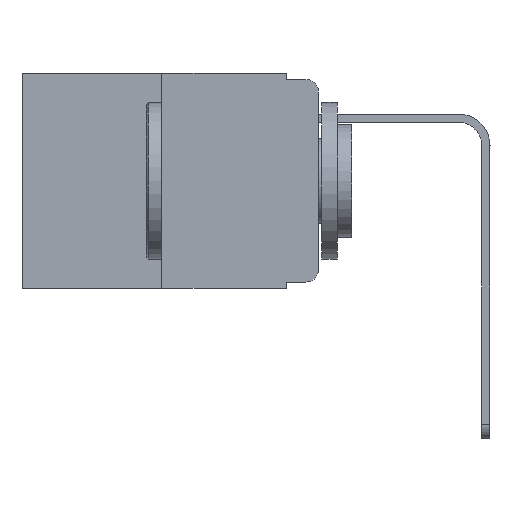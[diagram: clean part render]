
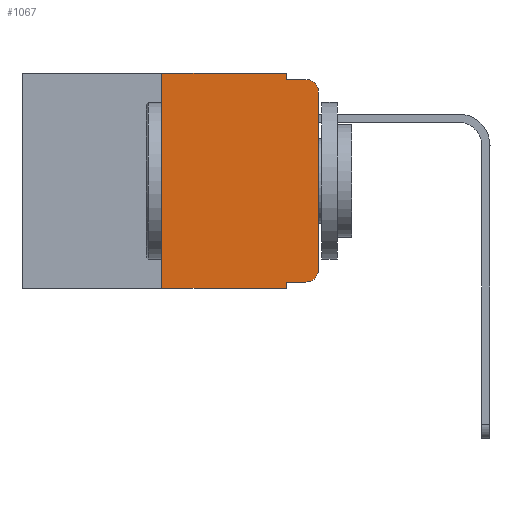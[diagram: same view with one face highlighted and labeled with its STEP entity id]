
A CAD part, left-side view. The second image highlights one B-rep face of the part: STEP entity #1067.
In plain terms, the highlighted planar face has unit normal (-1, 0, 0).
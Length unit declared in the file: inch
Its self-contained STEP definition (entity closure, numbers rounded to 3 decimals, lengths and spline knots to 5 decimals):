
#223 = CARTESIAN_POINT ( 'NONE',  ( 0., 0.051, 0. ) ) ;
#429 = DIRECTION ( 'NONE',  ( 0., 0., 1. ) ) ;
#489 = ORIENTED_EDGE ( 'NONE', *, *, #8777, .T. ) ;
#561 = DIRECTION ( 'NONE',  ( 0., -1., 0. ) ) ;
#603 = VERTEX_POINT ( 'NONE', #2960 ) ;
#658 = DIRECTION ( 'NONE',  ( 0., 0., -1. ) ) ;
#735 = CARTESIAN_POINT ( 'NONE',  ( 0., 0.051, -0.333 ) ) ;
#799 = EDGE_CURVE ( 'NONE', #10643, #1818, #5035, .T. ) ;
#955 = ORIENTED_EDGE ( 'NONE', *, *, #12084, .T. ) ;
#992 = LINE ( 'NONE', #735, #4520 ) ;
#1026 = CARTESIAN_POINT ( 'NONE',  ( 0., 0.02, -0.313 ) ) ;
#1067 = ADVANCED_FACE ( 'NONE', ( #10304 ), #7958, .F. ) ;
#1506 = EDGE_LOOP ( 'NONE', ( #489, #3924, #12947, #4434, #7880, #2469, #955, #7709, #5813, #2844 ) ) ;
#1687 = EDGE_CURVE ( 'NONE', #11537, #8962, #7487, .T. ) ;
#1818 = VERTEX_POINT ( 'NONE', #3817 ) ;
#2043 = DIRECTION ( 'NONE',  ( 0., 0., -1. ) ) ;
#2469 = ORIENTED_EDGE ( 'NONE', *, *, #799, .F. ) ;
#2681 = AXIS2_PLACEMENT_3D ( 'NONE', #11666, #5864, #658 ) ;
#2844 = ORIENTED_EDGE ( 'NONE', *, *, #12909, .T. ) ;
#2897 = DIRECTION ( 'NONE',  ( 0., 0., -1. ) ) ;
#2943 = CARTESIAN_POINT ( 'NONE',  ( 0., 0.473, 0. ) ) ;
#2946 = CARTESIAN_POINT ( 'NONE',  ( 0., 0.473, 0. ) ) ;
#2960 = CARTESIAN_POINT ( 'NONE',  ( 0., 0.051, -0.01 ) ) ;
#3241 = CARTESIAN_POINT ( 'NONE',  ( 0., 0., -0.03 ) ) ;
#3251 = DIRECTION ( 'NONE',  ( -1., 0., 0. ) ) ;
#3274 = LINE ( 'NONE', #10098, #12647 ) ;
#3314 = CARTESIAN_POINT ( 'NONE',  ( 0., 0.051, -0.333 ) ) ;
#3402 = CARTESIAN_POINT ( 'NONE',  ( 0., 0.02, -0.01 ) ) ;
#3679 = DIRECTION ( 'NONE',  ( 0., -1., 0. ) ) ;
#3725 = CARTESIAN_POINT ( 'NONE',  ( 0., 0.051, -0.343 ) ) ;
#3817 = CARTESIAN_POINT ( 'NONE',  ( 0., 0.25, 0. ) ) ;
#3924 = ORIENTED_EDGE ( 'NONE', *, *, #1687, .T. ) ;
#4434 = ORIENTED_EDGE ( 'NONE', *, *, #4542, .F. ) ;
#4520 = VECTOR ( 'NONE', #12689, 39.37008 ) ;
#4542 = EDGE_CURVE ( 'NONE', #12334, #603, #10764, .T. ) ;
#4618 = CIRCLE ( 'NONE', #10205, 0.02 ) ;
#4820 = DIRECTION ( 'NONE',  ( 0., -1., 0. ) ) ;
#4946 = VECTOR ( 'NONE', #561, 39.37008 ) ;
#4997 = EDGE_CURVE ( 'NONE', #8837, #7947, #992, .T. ) ;
#5035 = LINE ( 'NONE', #5432, #12028 ) ;
#5089 = VECTOR ( 'NONE', #4820, 39.37008 ) ;
#5432 = CARTESIAN_POINT ( 'NONE',  ( 0., 0.25, 0. ) ) ;
#5601 = DIRECTION ( 'NONE',  ( 0., 0., -1. ) ) ;
#5721 = LINE ( 'NONE', #6640, #4946 ) ;
#5738 = EDGE_CURVE ( 'NONE', #8837, #12107, #11523, .T. ) ;
#5758 = DIRECTION ( 'NONE',  ( 0., 0., 1. ) ) ;
#5813 = ORIENTED_EDGE ( 'NONE', *, *, #4997, .T. ) ;
#5864 = DIRECTION ( 'NONE',  ( -1., 0., 0. ) ) ;
#6640 = CARTESIAN_POINT ( 'NONE',  ( 0., 0.051, -0.01 ) ) ;
#6788 = CARTESIAN_POINT ( 'NONE',  ( 0., 0.473, -0.343 ) ) ;
#7487 = CIRCLE ( 'NONE', #2681, 0.02 ) ;
#7550 = EDGE_CURVE ( 'NONE', #1818, #12334, #10692, .T. ) ;
#7598 = LINE ( 'NONE', #6788, #10877 ) ;
#7709 = ORIENTED_EDGE ( 'NONE', *, *, #5738, .F. ) ;
#7880 = ORIENTED_EDGE ( 'NONE', *, *, #7550, .F. ) ;
#7947 = VERTEX_POINT ( 'NONE', #12554 ) ;
#7958 = PLANE ( 'NONE',  #8747 ) ;
#8747 = AXIS2_PLACEMENT_3D ( 'NONE', #2943, #8911, #2897 ) ;
#8777 = EDGE_CURVE ( 'NONE', #12714, #11537, #3274, .T. ) ;
#8837 = VERTEX_POINT ( 'NONE', #3314 ) ;
#8890 = VECTOR ( 'NONE', #11678, 39.37008 ) ;
#8911 = DIRECTION ( 'NONE',  ( 1., 0., 0. ) ) ;
#8962 = VERTEX_POINT ( 'NONE', #3402 ) ;
#10098 = CARTESIAN_POINT ( 'NONE',  ( 0., 0., 0. ) ) ;
#10205 = AXIS2_PLACEMENT_3D ( 'NONE', #1026, #3251, #2043 ) ;
#10304 = FACE_OUTER_BOUND ( 'NONE', #1506, .T. ) ;
#10440 = VECTOR ( 'NONE', #5601, 39.37008 ) ;
#10643 = VERTEX_POINT ( 'NONE', #12695 ) ;
#10692 = LINE ( 'NONE', #2946, #5089 ) ;
#10764 = LINE ( 'NONE', #12558, #10440 ) ;
#10877 = VECTOR ( 'NONE', #3679, 39.37008 ) ;
#11523 = LINE ( 'NONE', #12715, #8890 ) ;
#11537 = VERTEX_POINT ( 'NONE', #3241 ) ;
#11666 = CARTESIAN_POINT ( 'NONE',  ( 0., 0.02, -0.03 ) ) ;
#11678 = DIRECTION ( 'NONE',  ( 0., 0., -1. ) ) ;
#11828 = CARTESIAN_POINT ( 'NONE',  ( 0., 0., -0.313 ) ) ;
#12028 = VECTOR ( 'NONE', #429, 39.37008 ) ;
#12084 = EDGE_CURVE ( 'NONE', #10643, #12107, #7598, .T. ) ;
#12107 = VERTEX_POINT ( 'NONE', #3725 ) ;
#12334 = VERTEX_POINT ( 'NONE', #223 ) ;
#12554 = CARTESIAN_POINT ( 'NONE',  ( 0., 0.02, -0.333 ) ) ;
#12558 = CARTESIAN_POINT ( 'NONE',  ( 0., 0.051, 0. ) ) ;
#12618 = EDGE_CURVE ( 'NONE', #603, #8962, #5721, .T. ) ;
#12647 = VECTOR ( 'NONE', #5758, 39.37008 ) ;
#12689 = DIRECTION ( 'NONE',  ( 0., -1., 0. ) ) ;
#12695 = CARTESIAN_POINT ( 'NONE',  ( 0., 0.25, -0.343 ) ) ;
#12714 = VERTEX_POINT ( 'NONE', #11828 ) ;
#12715 = CARTESIAN_POINT ( 'NONE',  ( 0., 0.051, 0. ) ) ;
#12909 = EDGE_CURVE ( 'NONE', #7947, #12714, #4618, .T. ) ;
#12947 = ORIENTED_EDGE ( 'NONE', *, *, #12618, .F. ) ;
